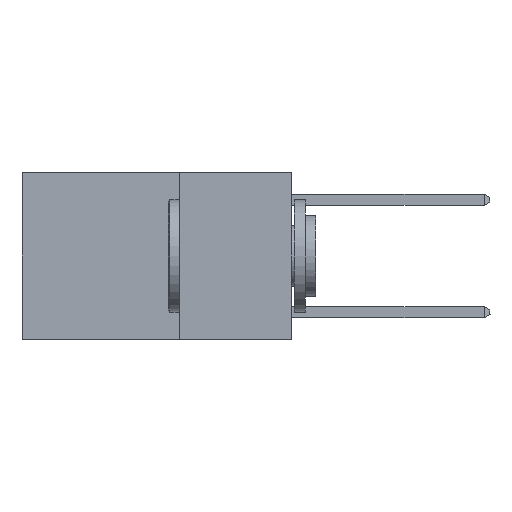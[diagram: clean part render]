
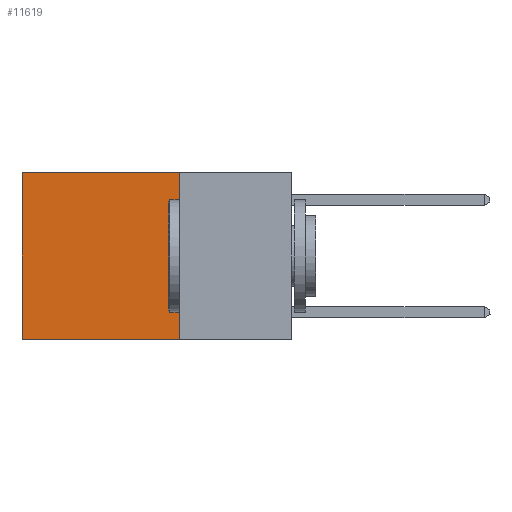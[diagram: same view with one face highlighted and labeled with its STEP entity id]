
A CAD part, left-side view. The second image highlights one B-rep face of the part: STEP entity #11619.
In plain terms, the highlighted planar face has unit normal (-1, 0, 0).
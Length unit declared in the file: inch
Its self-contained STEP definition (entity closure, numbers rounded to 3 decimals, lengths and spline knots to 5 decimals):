
#146 = ORIENTED_EDGE ( 'NONE', *, *, #10978, .T. ) ;
#769 = CARTESIAN_POINT ( 'NONE',  ( 0.2625, 0.6, -0.37 ) ) ;
#1052 = CARTESIAN_POINT ( 'NONE',  ( 0.2625, 0.25, -0.37 ) ) ;
#2356 = LINE ( 'NONE', #8738, #5282 ) ;
#3239 = ORIENTED_EDGE ( 'NONE', *, *, #10327, .F. ) ;
#4478 = ORIENTED_EDGE ( 'NONE', *, *, #20886, .T. ) ;
#5282 = VECTOR ( 'NONE', #10837, 39.37008 ) ;
#5424 = EDGE_CURVE ( 'NONE', #18821, #21975, #23617, .T. ) ;
#5495 = VERTEX_POINT ( 'NONE', #769 ) ;
#5874 = CARTESIAN_POINT ( 'NONE',  ( 0.2625, 0.25, 0. ) ) ;
#7306 = LINE ( 'NONE', #5874, #23538 ) ;
#8066 = FACE_OUTER_BOUND ( 'NONE', #16439, .T. ) ;
#8738 = CARTESIAN_POINT ( 'NONE',  ( 0.2625, 0.25, -0.37 ) ) ;
#10327 = EDGE_CURVE ( 'NONE', #21975, #5495, #2356, .T. ) ;
#10837 = DIRECTION ( 'NONE',  ( 0., 1., 0. ) ) ;
#10978 = EDGE_CURVE ( 'NONE', #18821, #17956, #7306, .T. ) ;
#11353 = VECTOR ( 'NONE', #23597, 39.37008 ) ;
#11619 = ADVANCED_FACE ( 'NONE', ( #8066 ), #27285, .F. ) ;
#12280 = DIRECTION ( 'NONE',  ( 0., 1., 0. ) ) ;
#13148 = CARTESIAN_POINT ( 'NONE',  ( 0.2625, 0.25, 0. ) ) ;
#14616 = DIRECTION ( 'NONE',  ( 1., 0., 0. ) ) ;
#15193 = ORIENTED_EDGE ( 'NONE', *, *, #5424, .F. ) ;
#15406 = VECTOR ( 'NONE', #17748, 39.37008 ) ;
#15646 = LINE ( 'NONE', #24154, #11353 ) ;
#16439 = EDGE_LOOP ( 'NONE', ( #4478, #3239, #15193, #146 ) ) ;
#16696 = CARTESIAN_POINT ( 'NONE',  ( 0.2625, 0.25, 0. ) ) ;
#17748 = DIRECTION ( 'NONE',  ( 0., 0., -1. ) ) ;
#17956 = VERTEX_POINT ( 'NONE', #25980 ) ;
#18667 = DIRECTION ( 'NONE',  ( 0., 0., -1. ) ) ;
#18685 = AXIS2_PLACEMENT_3D ( 'NONE', #16696, #14616, #18667 ) ;
#18821 = VERTEX_POINT ( 'NONE', #25786 ) ;
#20886 = EDGE_CURVE ( 'NONE', #17956, #5495, #15646, .T. ) ;
#21975 = VERTEX_POINT ( 'NONE', #1052 ) ;
#23538 = VECTOR ( 'NONE', #12280, 39.37008 ) ;
#23597 = DIRECTION ( 'NONE',  ( 0., 0., -1. ) ) ;
#23617 = LINE ( 'NONE', #13148, #15406 ) ;
#24154 = CARTESIAN_POINT ( 'NONE',  ( 0.2625, 0.6, 0. ) ) ;
#25786 = CARTESIAN_POINT ( 'NONE',  ( 0.2625, 0.25, 0. ) ) ;
#25980 = CARTESIAN_POINT ( 'NONE',  ( 0.2625, 0.6, 0. ) ) ;
#27285 = PLANE ( 'NONE',  #18685 ) ;
